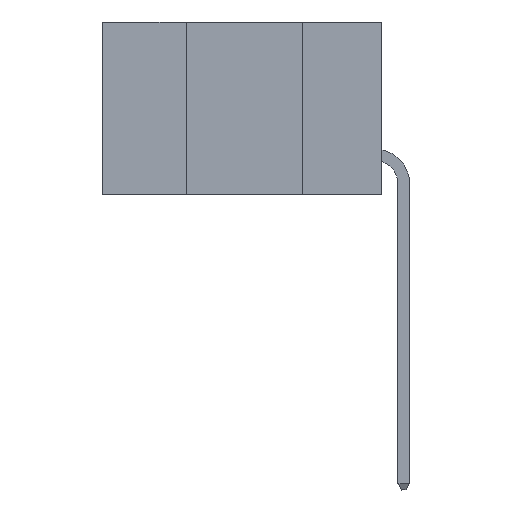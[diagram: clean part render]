
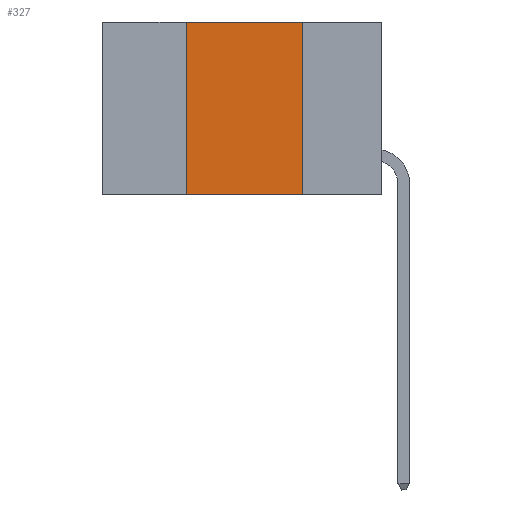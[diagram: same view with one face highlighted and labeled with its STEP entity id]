
A CAD part, left-side view. The second image highlights one B-rep face of the part: STEP entity #327.
In plain terms, the highlighted planar face has unit normal (-1, 0, 0).
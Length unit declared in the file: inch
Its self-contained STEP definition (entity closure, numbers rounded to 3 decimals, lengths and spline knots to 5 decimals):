
#327 = ADVANCED_FACE ( 'NONE', ( #9127 ), #14970, .F. ) ;
#1825 = VECTOR ( 'NONE', #16105, 39.37008 ) ;
#2051 = DIRECTION ( 'NONE',  ( 0., 0., 1. ) ) ;
#2170 = EDGE_CURVE ( 'NONE', #17866, #17892, #18495, .T. ) ;
#2845 = CARTESIAN_POINT ( 'NONE',  ( 0., 0.6, -0.37 ) ) ;
#2995 = LINE ( 'NONE', #23643, #21944 ) ;
#3853 = VECTOR ( 'NONE', #2051, 39.37008 ) ;
#4086 = VECTOR ( 'NONE', #21379, 39.37008 ) ;
#5592 = CARTESIAN_POINT ( 'NONE',  ( 0., 0.17, -0.37 ) ) ;
#5866 = CARTESIAN_POINT ( 'NONE',  ( 0., 0.42, 0. ) ) ;
#5945 = DIRECTION ( 'NONE',  ( 1., 0., 0. ) ) ;
#6219 = CARTESIAN_POINT ( 'NONE',  ( 0., 0.17, 0. ) ) ;
#6703 = EDGE_LOOP ( 'NONE', ( #21006, #21342, #7813, #14124 ) ) ;
#7097 = VERTEX_POINT ( 'NONE', #17840 ) ;
#7533 = LINE ( 'NONE', #6219, #1825 ) ;
#7813 = ORIENTED_EDGE ( 'NONE', *, *, #2170, .F. ) ;
#8924 = EDGE_CURVE ( 'NONE', #17892, #7097, #2995, .T. ) ;
#9127 = FACE_OUTER_BOUND ( 'NONE', #6703, .T. ) ;
#11449 = CARTESIAN_POINT ( 'NONE',  ( 0., 0.6, 0. ) ) ;
#13323 = EDGE_CURVE ( 'NONE', #7097, #14097, #7533, .T. ) ;
#13481 = EDGE_CURVE ( 'NONE', #17866, #14097, #13862, .T. ) ;
#13862 = LINE ( 'NONE', #2845, #4086 ) ;
#14097 = VERTEX_POINT ( 'NONE', #5592 ) ;
#14124 = ORIENTED_EDGE ( 'NONE', *, *, #13481, .T. ) ;
#14970 = PLANE ( 'NONE',  #16045 ) ;
#16045 = AXIS2_PLACEMENT_3D ( 'NONE', #11449, #5945, #16863 ) ;
#16105 = DIRECTION ( 'NONE',  ( 0., 0., -1. ) ) ;
#16863 = DIRECTION ( 'NONE',  ( 0., 0., -1. ) ) ;
#17840 = CARTESIAN_POINT ( 'NONE',  ( 0., 0.17, 0. ) ) ;
#17866 = VERTEX_POINT ( 'NONE', #21641 ) ;
#17892 = VERTEX_POINT ( 'NONE', #19955 ) ;
#18495 = LINE ( 'NONE', #5866, #3853 ) ;
#19955 = CARTESIAN_POINT ( 'NONE',  ( 0., 0.42, 0. ) ) ;
#21006 = ORIENTED_EDGE ( 'NONE', *, *, #13323, .F. ) ;
#21342 = ORIENTED_EDGE ( 'NONE', *, *, #8924, .F. ) ;
#21379 = DIRECTION ( 'NONE',  ( 0., -1., 0. ) ) ;
#21641 = CARTESIAN_POINT ( 'NONE',  ( 0., 0.42, -0.37 ) ) ;
#21944 = VECTOR ( 'NONE', #23564, 39.37008 ) ;
#23564 = DIRECTION ( 'NONE',  ( 0., -1., 0. ) ) ;
#23643 = CARTESIAN_POINT ( 'NONE',  ( 0., 0.6, 0. ) ) ;
